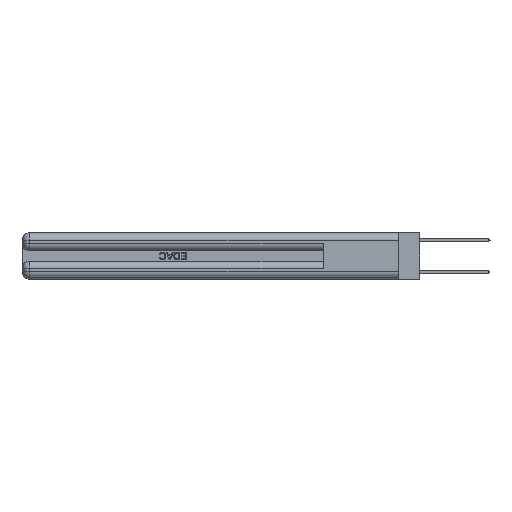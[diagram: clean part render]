
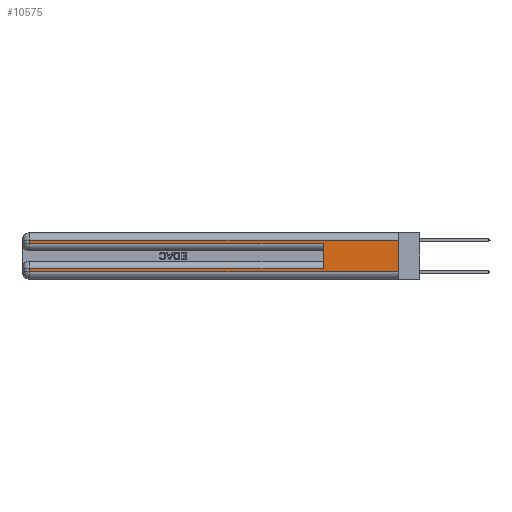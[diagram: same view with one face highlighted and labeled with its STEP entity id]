
A CAD part, left-side view. The second image highlights one B-rep face of the part: STEP entity #10575.
In plain terms, the highlighted planar face has unit normal (-1, 0, 0).
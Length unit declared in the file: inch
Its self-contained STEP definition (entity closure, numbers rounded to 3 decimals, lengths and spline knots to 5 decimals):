
#786 = LINE ( 'NONE', #2051, #14451 ) ;
#995 = DIRECTION ( 'NONE',  ( 0., -1., 0. ) ) ;
#1295 = VECTOR ( 'NONE', #19499, 39.37008 ) ;
#1409 = VERTEX_POINT ( 'NONE', #12352 ) ;
#1440 = LINE ( 'NONE', #28746, #15126 ) ;
#2051 = CARTESIAN_POINT ( 'NONE',  ( 0., 0., 0.37 ) ) ;
#2053 = VECTOR ( 'NONE', #15074, 39.37008 ) ;
#2567 = EDGE_CURVE ( 'NONE', #1409, #30750, #14979, .T. ) ;
#3125 = EDGE_CURVE ( 'NONE', #6163, #32678, #5961, .T. ) ;
#3429 = CARTESIAN_POINT ( 'NONE',  ( 0., 0., 0.31 ) ) ;
#3640 = CARTESIAN_POINT ( 'NONE',  ( 0., 0., 0.06 ) ) ;
#3708 = EDGE_CURVE ( 'NONE', #22611, #10289, #786, .T. ) ;
#4794 = DIRECTION ( 'NONE',  ( 0., 0., -1. ) ) ;
#5643 = CARTESIAN_POINT ( 'NONE',  ( 0., 2.94, 0.06 ) ) ;
#5961 = LINE ( 'NONE', #27425, #18794 ) ;
#6163 = VERTEX_POINT ( 'NONE', #10109 ) ;
#6180 = DIRECTION ( 'NONE',  ( 0., 1., 0. ) ) ;
#7040 = VECTOR ( 'NONE', #6180, 39.37008 ) ;
#7924 = ORIENTED_EDGE ( 'NONE', *, *, #19806, .T. ) ;
#7929 = ORIENTED_EDGE ( 'NONE', *, *, #9336, .F. ) ;
#8009 = CARTESIAN_POINT ( 'NONE',  ( 0., 0.6, 0.285 ) ) ;
#8594 = LINE ( 'NONE', #9220, #29480 ) ;
#9220 = CARTESIAN_POINT ( 'NONE',  ( 0., 0., 0.06 ) ) ;
#9336 = EDGE_CURVE ( 'NONE', #1409, #32678, #32205, .T. ) ;
#9884 = FACE_OUTER_BOUND ( 'NONE', #16559, .T. ) ;
#9989 = CARTESIAN_POINT ( 'NONE',  ( 0., 0.6, 0.145 ) ) ;
#10067 = AXIS2_PLACEMENT_3D ( 'NONE', #31904, #34648, #18325 ) ;
#10109 = CARTESIAN_POINT ( 'NONE',  ( 0., 2.94, 0.285 ) ) ;
#10289 = VERTEX_POINT ( 'NONE', #3640 ) ;
#10575 = ADVANCED_FACE ( 'NONE', ( #9884 ), #18212, .F. ) ;
#11330 = CARTESIAN_POINT ( 'NONE',  ( 0., 0., 0.085 ) ) ;
#12352 = CARTESIAN_POINT ( 'NONE',  ( 0., 0.6, 0.085 ) ) ;
#12732 = DIRECTION ( 'NONE',  ( 0., 0., 1. ) ) ;
#12839 = ORIENTED_EDGE ( 'NONE', *, *, #3708, .F. ) ;
#13126 = CARTESIAN_POINT ( 'NONE',  ( 0., 2.94, 0.31 ) ) ;
#14451 = VECTOR ( 'NONE', #4794, 39.37008 ) ;
#14979 = LINE ( 'NONE', #11330, #1295 ) ;
#15074 = DIRECTION ( 'NONE',  ( 0., 0., -1. ) ) ;
#15126 = VECTOR ( 'NONE', #31522, 39.37008 ) ;
#16559 = EDGE_LOOP ( 'NONE', ( #12839, #32008, #32583, #25860, #7929, #25850, #7924, #31510 ) ) ;
#16875 = VERTEX_POINT ( 'NONE', #5643 ) ;
#18212 = PLANE ( 'NONE',  #10067 ) ;
#18325 = DIRECTION ( 'NONE',  ( 0., 0., -1. ) ) ;
#18794 = VECTOR ( 'NONE', #33029, 39.37008 ) ;
#19499 = DIRECTION ( 'NONE',  ( 0., 1., 0. ) ) ;
#19806 = EDGE_CURVE ( 'NONE', #30750, #16875, #1440, .T. ) ;
#22296 = CARTESIAN_POINT ( 'NONE',  ( 0., 2.94, 0.37 ) ) ;
#22363 = EDGE_CURVE ( 'NONE', #16875, #10289, #8594, .T. ) ;
#22611 = VERTEX_POINT ( 'NONE', #34868 ) ;
#25850 = ORIENTED_EDGE ( 'NONE', *, *, #2567, .T. ) ;
#25860 = ORIENTED_EDGE ( 'NONE', *, *, #3125, .T. ) ;
#25951 = EDGE_CURVE ( 'NONE', #22611, #27058, #30535, .T. ) ;
#27058 = VERTEX_POINT ( 'NONE', #13126 ) ;
#27425 = CARTESIAN_POINT ( 'NONE',  ( 0., 0., 0.285 ) ) ;
#28513 = LINE ( 'NONE', #22296, #2053 ) ;
#28746 = CARTESIAN_POINT ( 'NONE',  ( 0., 2.94, 0.37 ) ) ;
#29480 = VECTOR ( 'NONE', #995, 39.37008 ) ;
#30310 = EDGE_CURVE ( 'NONE', #27058, #6163, #28513, .T. ) ;
#30535 = LINE ( 'NONE', #3429, #7040 ) ;
#30750 = VERTEX_POINT ( 'NONE', #35346 ) ;
#31345 = VECTOR ( 'NONE', #12732, 39.37008 ) ;
#31510 = ORIENTED_EDGE ( 'NONE', *, *, #22363, .T. ) ;
#31522 = DIRECTION ( 'NONE',  ( 0., 0., -1. ) ) ;
#31904 = CARTESIAN_POINT ( 'NONE',  ( 0., 0., 0.37 ) ) ;
#32008 = ORIENTED_EDGE ( 'NONE', *, *, #25951, .T. ) ;
#32205 = LINE ( 'NONE', #9989, #31345 ) ;
#32583 = ORIENTED_EDGE ( 'NONE', *, *, #30310, .T. ) ;
#32678 = VERTEX_POINT ( 'NONE', #8009 ) ;
#33029 = DIRECTION ( 'NONE',  ( 0., -1., 0. ) ) ;
#34648 = DIRECTION ( 'NONE',  ( 1., 0., 0. ) ) ;
#34868 = CARTESIAN_POINT ( 'NONE',  ( 0., 0., 0.31 ) ) ;
#35346 = CARTESIAN_POINT ( 'NONE',  ( 0., 2.94, 0.085 ) ) ;
